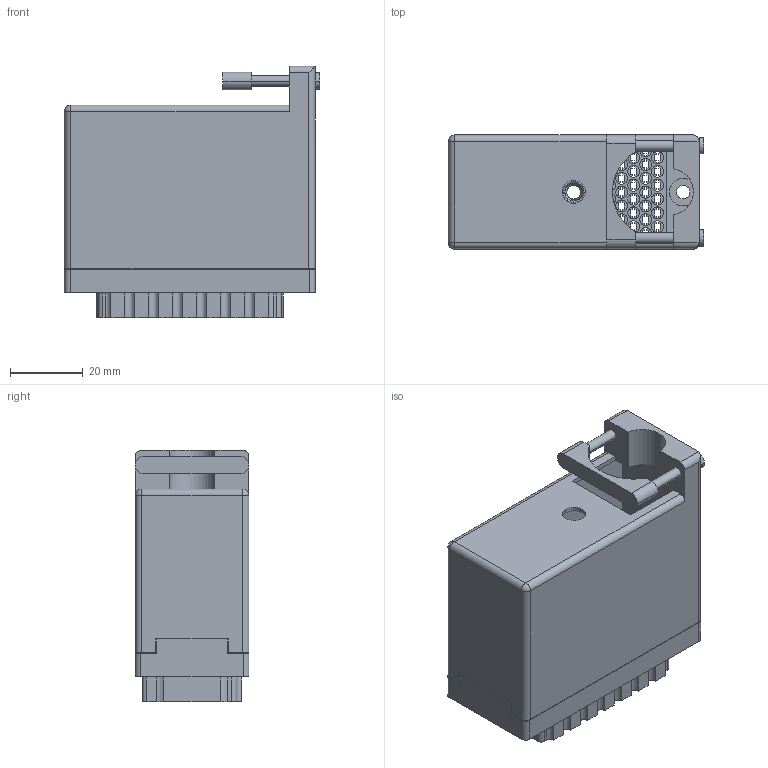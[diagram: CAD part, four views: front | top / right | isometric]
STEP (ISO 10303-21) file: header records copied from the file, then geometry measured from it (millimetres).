
FILE_DESCRIPTION (( 'STEP AP203' ), '1' );
FILE_NAME ('516-090-000-266.STEP', '2020-03-06T16:23:18', ( '' ), ( '' ), 'SwSTEP 2.0', 'SolidWorks 2016', '' );
FILE_SCHEMA (( 'CONFIG_CONTROL_DESIGN' ));
Length unit declared in the file: inch
Products named in the file (4): 516-230-001_Metal - 090 Top Entry; 516 Part Receptacle_090; 516-252-095-100; 516-090-000-266
Assembly tree (3 placements, depth 2):
  516-090-000-266
    516 Part Receptacle_090
    516-230-001_Metal - 090 Top Entry
    516-252-095-100
Bounding box: 70.31 x 31.34 x 69.24 mm (x, y, z)
Volume: 35203.2 mm3; surface area: 52258.8 mm2
Topology: 3 solids, 3 shells, 2038 faces, 6023 edges, 4007 vertices
Faces by surface type: plane 1419, cylinder 599, cone 12, bspline 6, sphere 2
Entity records: 70782 total; most frequent: CARTESIAN_POINT 14114, ORIENTED_EDGE 12042, DIRECTION 11592, EDGE_CURVE 6021, LINE 4418, VECTOR 4418, VERTEX_POINT 4007, AXIS2_PLACEMENT_3D 3587
